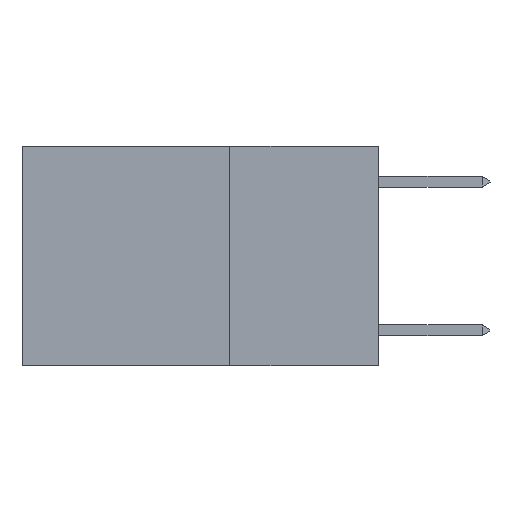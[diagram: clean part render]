
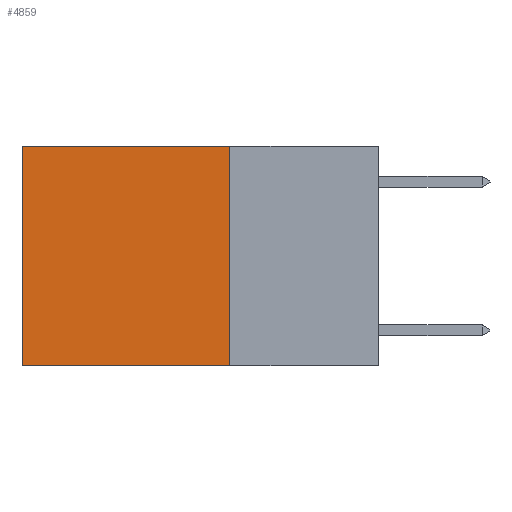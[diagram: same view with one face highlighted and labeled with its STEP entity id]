
A CAD part, left-side view. The second image highlights one B-rep face of the part: STEP entity #4859.
In plain terms, the highlighted planar face has unit normal (-1, 0, 0).
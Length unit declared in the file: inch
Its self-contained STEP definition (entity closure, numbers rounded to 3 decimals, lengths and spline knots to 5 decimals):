
#710 = VERTEX_POINT ( 'NONE', #2077 ) ;
#1353 = VERTEX_POINT ( 'NONE', #3531 ) ;
#1734 = DIRECTION ( 'NONE',  ( 1., 0., 0. ) ) ;
#2077 = CARTESIAN_POINT ( 'NONE',  ( 0.2625, 0.6, 0. ) ) ;
#2101 = ORIENTED_EDGE ( 'NONE', *, *, #15574, .F. ) ;
#2568 = EDGE_CURVE ( 'NONE', #710, #11669, #20541, .T. ) ;
#2801 = CARTESIAN_POINT ( 'NONE',  ( 0.2625, 0.6, 0. ) ) ;
#3292 = CARTESIAN_POINT ( 'NONE',  ( 0.2625, 0.25, -0.37 ) ) ;
#3451 = EDGE_LOOP ( 'NONE', ( #12341, #6297, #2101, #15009 ) ) ;
#3460 = FACE_OUTER_BOUND ( 'NONE', #3451, .T. ) ;
#3531 = CARTESIAN_POINT ( 'NONE',  ( 0.2625, 0.25, 0. ) ) ;
#4859 = ADVANCED_FACE ( 'NONE', ( #3460 ), #10496, .F. ) ;
#4891 = AXIS2_PLACEMENT_3D ( 'NONE', #17509, #1734, #11189 ) ;
#5136 = CARTESIAN_POINT ( 'NONE',  ( 0.2625, 0.6, -0.37 ) ) ;
#6215 = VECTOR ( 'NONE', #22412, 39.37008 ) ;
#6297 = ORIENTED_EDGE ( 'NONE', *, *, #16993, .F. ) ;
#6552 = VERTEX_POINT ( 'NONE', #11106 ) ;
#7915 = CARTESIAN_POINT ( 'NONE',  ( 0.2625, 0.25, 0. ) ) ;
#8503 = DIRECTION ( 'NONE',  ( 0., 1., 0. ) ) ;
#10496 = PLANE ( 'NONE',  #4891 ) ;
#11106 = CARTESIAN_POINT ( 'NONE',  ( 0.2625, 0.25, -0.37 ) ) ;
#11189 = DIRECTION ( 'NONE',  ( 0., 0., -1. ) ) ;
#11669 = VERTEX_POINT ( 'NONE', #5136 ) ;
#12341 = ORIENTED_EDGE ( 'NONE', *, *, #2568, .T. ) ;
#13163 = DIRECTION ( 'NONE',  ( 0., 0., -1. ) ) ;
#13880 = DIRECTION ( 'NONE',  ( 0., 1., 0. ) ) ;
#15009 = ORIENTED_EDGE ( 'NONE', *, *, #17961, .T. ) ;
#15574 = EDGE_CURVE ( 'NONE', #1353, #6552, #16657, .T. ) ;
#16657 = LINE ( 'NONE', #7915, #6215 ) ;
#16745 = VECTOR ( 'NONE', #13880, 39.37008 ) ;
#16792 = LINE ( 'NONE', #20721, #17661 ) ;
#16993 = EDGE_CURVE ( 'NONE', #6552, #11669, #22540, .T. ) ;
#17509 = CARTESIAN_POINT ( 'NONE',  ( 0.2625, 0.25, 0. ) ) ;
#17661 = VECTOR ( 'NONE', #8503, 39.37008 ) ;
#17961 = EDGE_CURVE ( 'NONE', #1353, #710, #16792, .T. ) ;
#20281 = VECTOR ( 'NONE', #13163, 39.37008 ) ;
#20541 = LINE ( 'NONE', #2801, #20281 ) ;
#20721 = CARTESIAN_POINT ( 'NONE',  ( 0.2625, 0.25, 0. ) ) ;
#22412 = DIRECTION ( 'NONE',  ( 0., 0., -1. ) ) ;
#22540 = LINE ( 'NONE', #3292, #16745 ) ;
